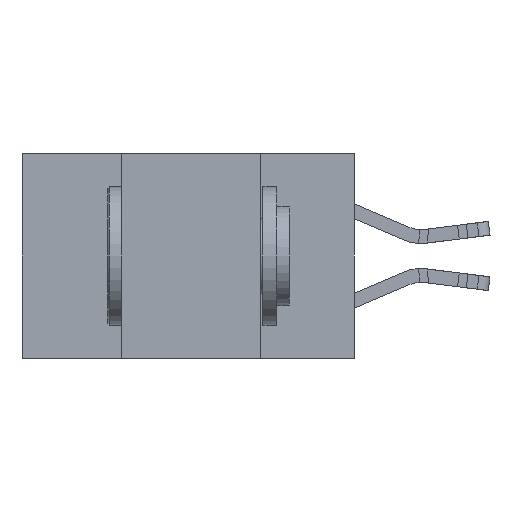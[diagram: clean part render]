
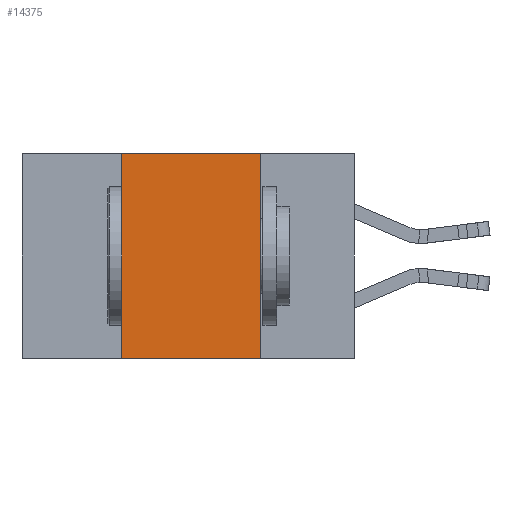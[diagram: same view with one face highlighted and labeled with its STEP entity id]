
A CAD part, left-side view. The second image highlights one B-rep face of the part: STEP entity #14375.
In plain terms, the highlighted planar face has unit normal (-1, 0, 0).
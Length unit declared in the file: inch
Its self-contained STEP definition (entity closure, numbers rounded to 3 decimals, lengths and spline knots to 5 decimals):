
#889 = VERTEX_POINT ( 'NONE', #17941 ) ;
#1420 = DIRECTION ( 'NONE',  ( 0., -1., 0. ) ) ;
#3116 = LINE ( 'NONE', #26972, #19531 ) ;
#3188 = CARTESIAN_POINT ( 'NONE',  ( 0., 0.42, -0.37 ) ) ;
#3831 = VECTOR ( 'NONE', #22804, 39.37008 ) ;
#3851 = PLANE ( 'NONE',  #11460 ) ;
#5771 = CARTESIAN_POINT ( 'NONE',  ( 0., 0.42, -0.37 ) ) ;
#6041 = FACE_OUTER_BOUND ( 'NONE', #27463, .T. ) ;
#7052 = EDGE_CURVE ( 'NONE', #21091, #24050, #23946, .T. ) ;
#8233 = DIRECTION ( 'NONE',  ( 1., 0., 0. ) ) ;
#9953 = ORIENTED_EDGE ( 'NONE', *, *, #17065, .F. ) ;
#11460 = AXIS2_PLACEMENT_3D ( 'NONE', #20961, #8233, #23059 ) ;
#11518 = DIRECTION ( 'NONE',  ( 0., -1., 0. ) ) ;
#12519 = VERTEX_POINT ( 'NONE', #3188 ) ;
#12634 = ORIENTED_EDGE ( 'NONE', *, *, #18479, .F. ) ;
#12745 = VECTOR ( 'NONE', #15255, 39.37008 ) ;
#14375 = ADVANCED_FACE ( 'NONE', ( #6041 ), #3851, .F. ) ;
#15053 = VECTOR ( 'NONE', #11518, 39.37008 ) ;
#15255 = DIRECTION ( 'NONE',  ( 0., 0., -1. ) ) ;
#15292 = LINE ( 'NONE', #5771, #3831 ) ;
#15403 = CARTESIAN_POINT ( 'NONE',  ( 0., 0.17, -0.37 ) ) ;
#17065 = EDGE_CURVE ( 'NONE', #12519, #889, #15292, .T. ) ;
#17941 = CARTESIAN_POINT ( 'NONE',  ( 0., 0.42, 0. ) ) ;
#18479 = EDGE_CURVE ( 'NONE', #889, #21091, #3116, .T. ) ;
#19167 = CARTESIAN_POINT ( 'NONE',  ( 0., 0.17, 0. ) ) ;
#19531 = VECTOR ( 'NONE', #1420, 39.37008 ) ;
#20220 = ORIENTED_EDGE ( 'NONE', *, *, #22716, .T. ) ;
#20961 = CARTESIAN_POINT ( 'NONE',  ( 0., 0.6, 0. ) ) ;
#21091 = VERTEX_POINT ( 'NONE', #19167 ) ;
#21130 = CARTESIAN_POINT ( 'NONE',  ( 0., 0.17, -0.37 ) ) ;
#21307 = LINE ( 'NONE', #26278, #15053 ) ;
#22529 = ORIENTED_EDGE ( 'NONE', *, *, #7052, .F. ) ;
#22716 = EDGE_CURVE ( 'NONE', #12519, #24050, #21307, .T. ) ;
#22804 = DIRECTION ( 'NONE',  ( 0., 0., 1. ) ) ;
#23059 = DIRECTION ( 'NONE',  ( 0., 0., -1. ) ) ;
#23946 = LINE ( 'NONE', #15403, #12745 ) ;
#24050 = VERTEX_POINT ( 'NONE', #21130 ) ;
#26278 = CARTESIAN_POINT ( 'NONE',  ( 0., 0.6, -0.37 ) ) ;
#26972 = CARTESIAN_POINT ( 'NONE',  ( 0., 0.6, 0. ) ) ;
#27463 = EDGE_LOOP ( 'NONE', ( #22529, #12634, #9953, #20220 ) ) ;
